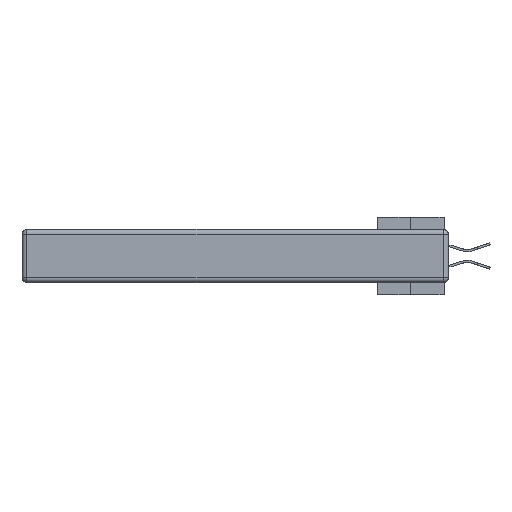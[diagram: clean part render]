
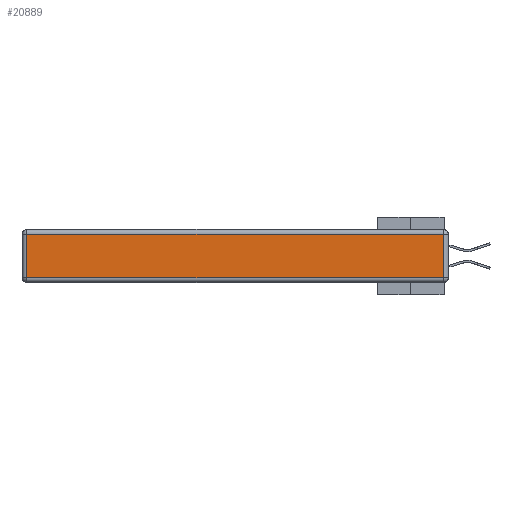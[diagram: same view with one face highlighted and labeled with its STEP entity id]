
A CAD part, left-side view. The second image highlights one B-rep face of the part: STEP entity #20889.
In plain terms, the highlighted planar face has unit normal (-1, 0, 0).
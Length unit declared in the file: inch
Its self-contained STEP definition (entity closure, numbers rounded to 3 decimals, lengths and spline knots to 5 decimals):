
#417 = ORIENTED_EDGE ( 'NONE', *, *, #23166, .T. ) ;
#705 = EDGE_CURVE ( 'NONE', #8414, #1809, #4803, .T. ) ;
#1326 = EDGE_CURVE ( 'NONE', #14824, #8414, #23588, .T. ) ;
#1809 = VERTEX_POINT ( 'NONE', #18490 ) ;
#2697 = DIRECTION ( 'NONE',  ( -1., 0., 0. ) ) ;
#2907 = LINE ( 'NONE', #20436, #32001 ) ;
#3179 = CARTESIAN_POINT ( 'NONE',  ( 0., 0.03, -0.313 ) ) ;
#4058 = EDGE_LOOP ( 'NONE', ( #8050, #21200, #11146, #417 ) ) ;
#4750 = DIRECTION ( 'NONE',  ( 0., 1., 0. ) ) ;
#4803 = LINE ( 'NONE', #6825, #14616 ) ;
#5328 = CARTESIAN_POINT ( 'NONE',  ( 0., 0., -0.343 ) ) ;
#5509 = VECTOR ( 'NONE', #4750, 39.37008 ) ;
#6825 = CARTESIAN_POINT ( 'NONE',  ( 0., 0.03, -0.343 ) ) ;
#7781 = VECTOR ( 'NONE', #24105, 39.37008 ) ;
#8050 = ORIENTED_EDGE ( 'NONE', *, *, #1326, .T. ) ;
#8414 = VERTEX_POINT ( 'NONE', #3179 ) ;
#11146 = ORIENTED_EDGE ( 'NONE', *, *, #32290, .T. ) ;
#12454 = CARTESIAN_POINT ( 'NONE',  ( 0., 2.72, -0.313 ) ) ;
#14616 = VECTOR ( 'NONE', #24411, 39.37008 ) ;
#14824 = VERTEX_POINT ( 'NONE', #12454 ) ;
#16055 = AXIS2_PLACEMENT_3D ( 'NONE', #5328, #2697, #21818 ) ;
#17136 = FACE_OUTER_BOUND ( 'NONE', #4058, .T. ) ;
#18340 = CARTESIAN_POINT ( 'NONE',  ( 0., 0., -0.313 ) ) ;
#18490 = CARTESIAN_POINT ( 'NONE',  ( 0., 0.03, -0.03 ) ) ;
#19993 = DIRECTION ( 'NONE',  ( 0., 0., -1. ) ) ;
#20436 = CARTESIAN_POINT ( 'NONE',  ( 0., 2.72, -0.343 ) ) ;
#20889 = ADVANCED_FACE ( 'NONE', ( #17136 ), #21697, .T. ) ;
#21200 = ORIENTED_EDGE ( 'NONE', *, *, #705, .T. ) ;
#21697 = PLANE ( 'NONE',  #16055 ) ;
#21818 = DIRECTION ( 'NONE',  ( 0., 0., 1. ) ) ;
#23166 = EDGE_CURVE ( 'NONE', #33698, #14824, #2907, .T. ) ;
#23588 = LINE ( 'NONE', #18340, #7781 ) ;
#24105 = DIRECTION ( 'NONE',  ( 0., -1., 0. ) ) ;
#24411 = DIRECTION ( 'NONE',  ( 0., 0., 1. ) ) ;
#25322 = CARTESIAN_POINT ( 'NONE',  ( 0., 2.72, -0.03 ) ) ;
#29482 = CARTESIAN_POINT ( 'NONE',  ( 0., 2.75, -0.03 ) ) ;
#32001 = VECTOR ( 'NONE', #19993, 39.37008 ) ;
#32290 = EDGE_CURVE ( 'NONE', #1809, #33698, #33713, .T. ) ;
#33698 = VERTEX_POINT ( 'NONE', #25322 ) ;
#33713 = LINE ( 'NONE', #29482, #5509 ) ;
